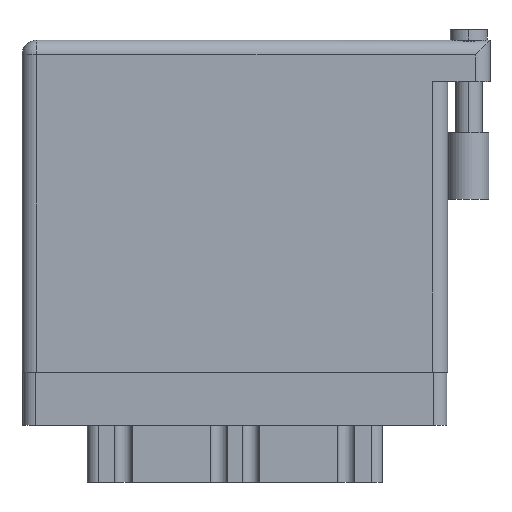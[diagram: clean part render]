
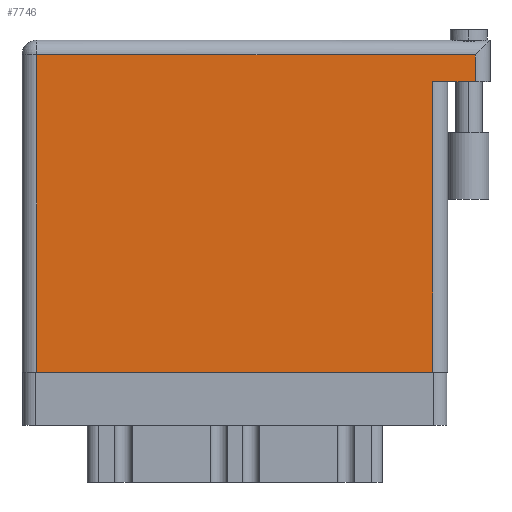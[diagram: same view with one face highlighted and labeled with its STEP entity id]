
A CAD part, front view. The second image highlights one B-rep face of the part: STEP entity #7746.
In plain terms, the highlighted face is planar.
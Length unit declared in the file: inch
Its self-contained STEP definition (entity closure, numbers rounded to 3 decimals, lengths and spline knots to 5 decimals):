
#45 = LINE ( 'NONE', #27067, #30159 ) ;
#230 = DIRECTION ( 'NONE',  ( -1., 0., 0. ) ) ;
#750 = ORIENTED_EDGE ( 'NONE', *, *, #24349, .T. ) ;
#1045 = DIRECTION ( 'NONE',  ( 0., 1., 0. ) ) ;
#1354 = DIRECTION ( 'NONE',  ( -1., 0., 0. ) ) ;
#1726 = AXIS2_PLACEMENT_3D ( 'NONE', #16125, #28001, #1354 ) ;
#1889 = EDGE_LOOP ( 'NONE', ( #16653, #750, #34559, #22752, #34207, #30434 ) ) ;
#2905 = VERTEX_POINT ( 'NONE', #33170 ) ;
#2992 = CARTESIAN_POINT ( 'NONE',  ( 0.07, 1.496, 0. ) ) ;
#3511 = FACE_OUTER_BOUND ( 'NONE', #1889, .T. ) ;
#5498 = EDGE_CURVE ( 'NONE', #15181, #32765, #17991, .T. ) ;
#5583 = VERTEX_POINT ( 'NONE', #18946 ) ;
#6511 = CARTESIAN_POINT ( 'NONE',  ( 0.07, 0., 0. ) ) ;
#7746 = ADVANCED_FACE ( 'NONE', ( #3511 ), #27807, .F. ) ;
#7990 = CARTESIAN_POINT ( 'NONE',  ( 2.138, 1.496, 0. ) ) ;
#8061 = DIRECTION ( 'NONE',  ( -1., 0., 0. ) ) ;
#10377 = LINE ( 'NONE', #33893, #33057 ) ;
#12965 = VERTEX_POINT ( 'NONE', #33506 ) ;
#13383 = EDGE_CURVE ( 'NONE', #5583, #12965, #13623, .T. ) ;
#13525 = CARTESIAN_POINT ( 'NONE',  ( 2.208, 1.369, 0. ) ) ;
#13623 = LINE ( 'NONE', #16718, #25626 ) ;
#15181 = VERTEX_POINT ( 'NONE', #34107 ) ;
#15267 = CARTESIAN_POINT ( 'NONE',  ( 2.138, 1.566, 0. ) ) ;
#15430 = VERTEX_POINT ( 'NONE', #2992 ) ;
#15673 = VECTOR ( 'NONE', #32756, 39.37008 ) ;
#16125 = CARTESIAN_POINT ( 'NONE',  ( 0., 1.566, 0. ) ) ;
#16653 = ORIENTED_EDGE ( 'NONE', *, *, #13383, .T. ) ;
#16718 = CARTESIAN_POINT ( 'NONE',  ( 0., 0., 0. ) ) ;
#17991 = LINE ( 'NONE', #15267, #26169 ) ;
#18365 = LINE ( 'NONE', #6511, #15673 ) ;
#18946 = CARTESIAN_POINT ( 'NONE',  ( 0.07, 0., 0. ) ) ;
#19165 = EDGE_CURVE ( 'NONE', #15181, #2905, #34701, .T. ) ;
#20998 = EDGE_CURVE ( 'NONE', #32765, #15430, #45, .T. ) ;
#21111 = DIRECTION ( 'NONE',  ( 0., 1., 0. ) ) ;
#22752 = ORIENTED_EDGE ( 'NONE', *, *, #5498, .T. ) ;
#24349 = EDGE_CURVE ( 'NONE', #12965, #2905, #10377, .T. ) ;
#25626 = VECTOR ( 'NONE', #36945, 39.37008 ) ;
#26169 = VECTOR ( 'NONE', #21111, 39.37008 ) ;
#27067 = CARTESIAN_POINT ( 'NONE',  ( 0., 1.496, 0. ) ) ;
#27807 = PLANE ( 'NONE',  #1726 ) ;
#28001 = DIRECTION ( 'NONE',  ( 0., 0., -1. ) ) ;
#30159 = VECTOR ( 'NONE', #230, 39.37008 ) ;
#30434 = ORIENTED_EDGE ( 'NONE', *, *, #31286, .T. ) ;
#31269 = VECTOR ( 'NONE', #8061, 39.37008 ) ;
#31286 = EDGE_CURVE ( 'NONE', #15430, #5583, #18365, .T. ) ;
#32756 = DIRECTION ( 'NONE',  ( 0., -1., 0. ) ) ;
#32765 = VERTEX_POINT ( 'NONE', #7990 ) ;
#33057 = VECTOR ( 'NONE', #1045, 39.37008 ) ;
#33170 = CARTESIAN_POINT ( 'NONE',  ( 1.938, 1.369, 0. ) ) ;
#33506 = CARTESIAN_POINT ( 'NONE',  ( 1.938, 0., 0. ) ) ;
#33893 = CARTESIAN_POINT ( 'NONE',  ( 1.938, 1.369, 0. ) ) ;
#34107 = CARTESIAN_POINT ( 'NONE',  ( 2.138, 1.369, 0. ) ) ;
#34207 = ORIENTED_EDGE ( 'NONE', *, *, #20998, .T. ) ;
#34559 = ORIENTED_EDGE ( 'NONE', *, *, #19165, .F. ) ;
#34701 = LINE ( 'NONE', #13525, #31269 ) ;
#36945 = DIRECTION ( 'NONE',  ( 1., 0., 0. ) ) ;
